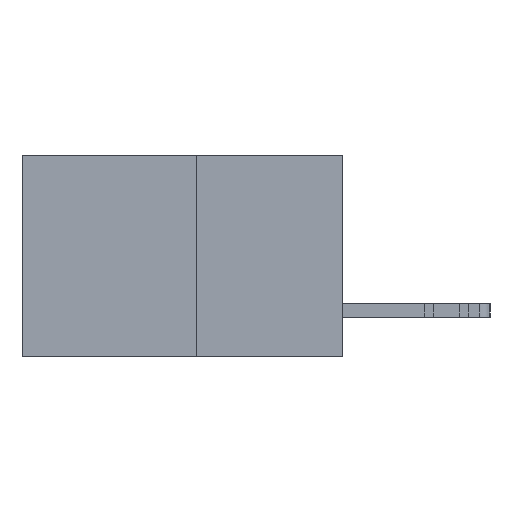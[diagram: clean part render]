
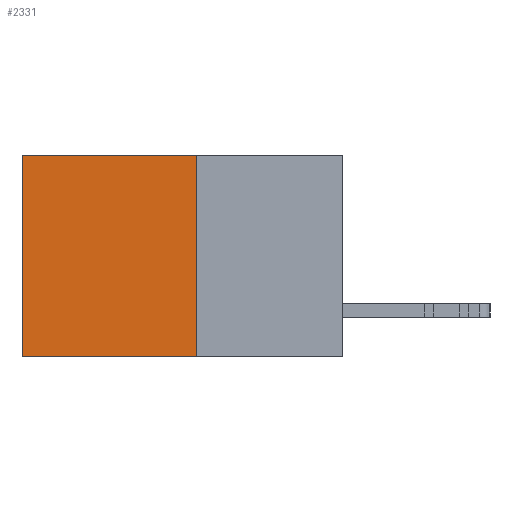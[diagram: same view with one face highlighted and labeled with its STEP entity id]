
A CAD part, left-side view. The second image highlights one B-rep face of the part: STEP entity #2331.
In plain terms, the highlighted planar face has unit normal (-1, 0, 0).
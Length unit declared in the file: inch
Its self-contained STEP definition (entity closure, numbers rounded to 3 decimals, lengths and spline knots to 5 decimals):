
#300 = CARTESIAN_POINT ( 'NONE',  ( 0.277, 0.59, 0. ) ) ;
#639 = EDGE_LOOP ( 'NONE', ( #23836, #24468, #1546, #24215 ) ) ;
#1546 = ORIENTED_EDGE ( 'NONE', *, *, #5731, .F. ) ;
#1603 = CARTESIAN_POINT ( 'NONE',  ( 0.277, 0.59, -0.37 ) ) ;
#2331 = ADVANCED_FACE ( 'NONE', ( #2902 ), #2949, .F. ) ;
#2902 = FACE_OUTER_BOUND ( 'NONE', #639, .T. ) ;
#2949 = PLANE ( 'NONE',  #23155 ) ;
#4423 = EDGE_CURVE ( 'NONE', #30667, #25756, #5827, .T. ) ;
#4985 = VECTOR ( 'NONE', #30713, 39.37008 ) ;
#5579 = DIRECTION ( 'NONE',  ( 1., 0., 0. ) ) ;
#5731 = EDGE_CURVE ( 'NONE', #16131, #30667, #28285, .T. ) ;
#5827 = LINE ( 'NONE', #8872, #32841 ) ;
#8716 = CARTESIAN_POINT ( 'NONE',  ( 0.277, 0.59, -0.37 ) ) ;
#8872 = CARTESIAN_POINT ( 'NONE',  ( 0.277, 0.27, -0.37 ) ) ;
#9938 = CARTESIAN_POINT ( 'NONE',  ( 0.277, 0.27, -0.37 ) ) ;
#12756 = LINE ( 'NONE', #17686, #4985 ) ;
#14845 = EDGE_CURVE ( 'NONE', #20662, #25756, #23680, .T. ) ;
#16131 = VERTEX_POINT ( 'NONE', #22230 ) ;
#17686 = CARTESIAN_POINT ( 'NONE',  ( 0.277, 0.27, 0. ) ) ;
#17752 = EDGE_CURVE ( 'NONE', #16131, #20662, #12756, .T. ) ;
#19305 = DIRECTION ( 'NONE',  ( 0., 1., 0. ) ) ;
#19656 = VECTOR ( 'NONE', #23005, 39.37008 ) ;
#19696 = CARTESIAN_POINT ( 'NONE',  ( 0.277, 0.27, -0.37 ) ) ;
#20662 = VERTEX_POINT ( 'NONE', #300 ) ;
#21275 = CARTESIAN_POINT ( 'NONE',  ( 0.277, 0.27, -0.37 ) ) ;
#22230 = CARTESIAN_POINT ( 'NONE',  ( 0.277, 0.27, 0. ) ) ;
#23005 = DIRECTION ( 'NONE',  ( 0., 0., -1. ) ) ;
#23155 = AXIS2_PLACEMENT_3D ( 'NONE', #21275, #5579, #23886 ) ;
#23680 = LINE ( 'NONE', #1603, #29790 ) ;
#23836 = ORIENTED_EDGE ( 'NONE', *, *, #14845, .T. ) ;
#23886 = DIRECTION ( 'NONE',  ( 0., 0., -1. ) ) ;
#24215 = ORIENTED_EDGE ( 'NONE', *, *, #17752, .T. ) ;
#24468 = ORIENTED_EDGE ( 'NONE', *, *, #4423, .F. ) ;
#25756 = VERTEX_POINT ( 'NONE', #8716 ) ;
#28285 = LINE ( 'NONE', #9938, #19656 ) ;
#29790 = VECTOR ( 'NONE', #30397, 39.37008 ) ;
#30397 = DIRECTION ( 'NONE',  ( 0., 0., -1. ) ) ;
#30667 = VERTEX_POINT ( 'NONE', #19696 ) ;
#30713 = DIRECTION ( 'NONE',  ( 0., 1., 0. ) ) ;
#32841 = VECTOR ( 'NONE', #19305, 39.37008 ) ;
